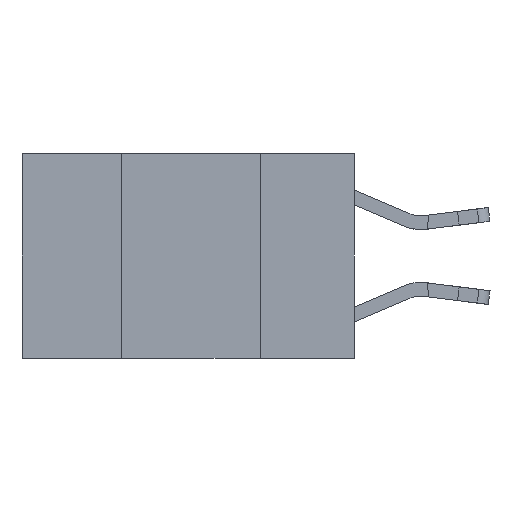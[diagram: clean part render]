
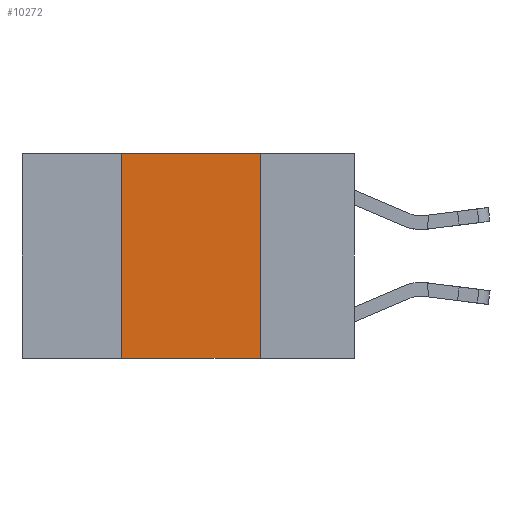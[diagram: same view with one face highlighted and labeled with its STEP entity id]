
A CAD part, left-side view. The second image highlights one B-rep face of the part: STEP entity #10272.
In plain terms, the highlighted planar face has unit normal (-1, 0, 0).
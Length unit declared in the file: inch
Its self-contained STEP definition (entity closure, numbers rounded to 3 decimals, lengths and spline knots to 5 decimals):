
#669 = LINE ( 'NONE', #15500, #8506 ) ;
#827 = VERTEX_POINT ( 'NONE', #9964 ) ;
#1461 = LINE ( 'NONE', #13292, #15356 ) ;
#2260 = ORIENTED_EDGE ( 'NONE', *, *, #10807, .F. ) ;
#2526 = EDGE_LOOP ( 'NONE', ( #14492, #7825, #2260, #2693 ) ) ;
#2693 = ORIENTED_EDGE ( 'NONE', *, *, #9002, .T. ) ;
#3171 = VERTEX_POINT ( 'NONE', #8902 ) ;
#3901 = DIRECTION ( 'NONE',  ( 0., -1., 0. ) ) ;
#4466 = CARTESIAN_POINT ( 'NONE',  ( 0., 0.42, 0. ) ) ;
#5280 = CARTESIAN_POINT ( 'NONE',  ( 0., 0.17, -0.37 ) ) ;
#6047 = AXIS2_PLACEMENT_3D ( 'NONE', #7546, #16794, #8933 ) ;
#6480 = CARTESIAN_POINT ( 'NONE',  ( 0., 0.42, 0. ) ) ;
#7017 = LINE ( 'NONE', #4466, #15312 ) ;
#7546 = CARTESIAN_POINT ( 'NONE',  ( 0., 0.6, 0. ) ) ;
#7825 = ORIENTED_EDGE ( 'NONE', *, *, #9249, .F. ) ;
#8506 = VECTOR ( 'NONE', #8953, 39.37008 ) ;
#8544 = VERTEX_POINT ( 'NONE', #6480 ) ;
#8902 = CARTESIAN_POINT ( 'NONE',  ( 0., 0.42, -0.37 ) ) ;
#8933 = DIRECTION ( 'NONE',  ( 0., 0., -1. ) ) ;
#8953 = DIRECTION ( 'NONE',  ( 0., 0., -1. ) ) ;
#9002 = EDGE_CURVE ( 'NONE', #3171, #14949, #15170, .T. ) ;
#9249 = EDGE_CURVE ( 'NONE', #8544, #827, #1461, .T. ) ;
#9964 = CARTESIAN_POINT ( 'NONE',  ( 0., 0.17, 0. ) ) ;
#10272 = ADVANCED_FACE ( 'NONE', ( #14122 ), #14197, .F. ) ;
#10807 = EDGE_CURVE ( 'NONE', #3171, #8544, #7017, .T. ) ;
#11549 = CARTESIAN_POINT ( 'NONE',  ( 0., 0.6, -0.37 ) ) ;
#11709 = EDGE_CURVE ( 'NONE', #827, #14949, #669, .T. ) ;
#13292 = CARTESIAN_POINT ( 'NONE',  ( 0., 0.6, 0. ) ) ;
#13863 = DIRECTION ( 'NONE',  ( 0., 0., 1. ) ) ;
#14122 = FACE_OUTER_BOUND ( 'NONE', #2526, .T. ) ;
#14197 = PLANE ( 'NONE',  #6047 ) ;
#14492 = ORIENTED_EDGE ( 'NONE', *, *, #11709, .F. ) ;
#14781 = VECTOR ( 'NONE', #15448, 39.37008 ) ;
#14949 = VERTEX_POINT ( 'NONE', #5280 ) ;
#15170 = LINE ( 'NONE', #11549, #14781 ) ;
#15312 = VECTOR ( 'NONE', #13863, 39.37008 ) ;
#15356 = VECTOR ( 'NONE', #3901, 39.37008 ) ;
#15448 = DIRECTION ( 'NONE',  ( 0., -1., 0. ) ) ;
#15500 = CARTESIAN_POINT ( 'NONE',  ( 0., 0.17, 0. ) ) ;
#16794 = DIRECTION ( 'NONE',  ( 1., 0., 0. ) ) ;
